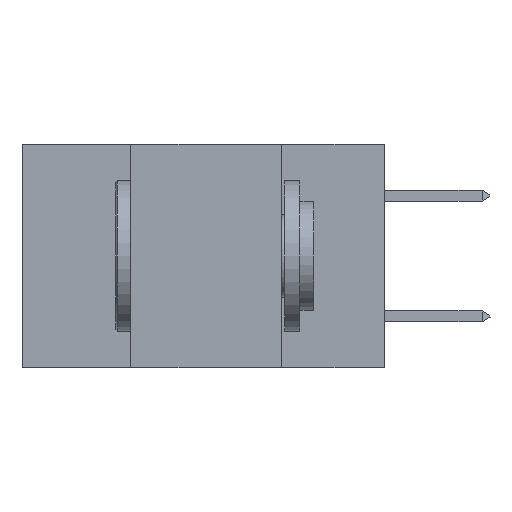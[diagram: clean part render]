
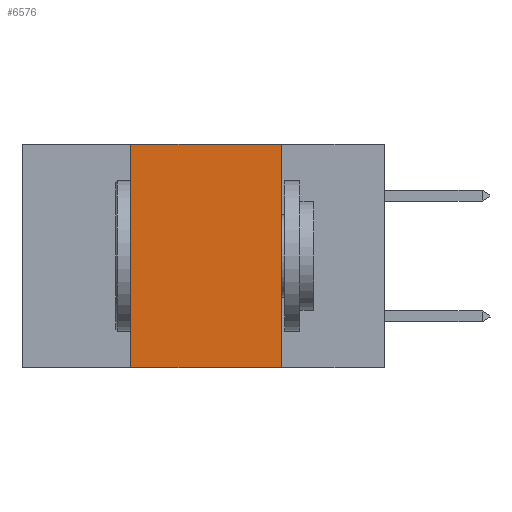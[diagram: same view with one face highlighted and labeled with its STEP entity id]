
A CAD part, left-side view. The second image highlights one B-rep face of the part: STEP entity #6576.
In plain terms, the highlighted planar face has unit normal (-1, 0, 0).
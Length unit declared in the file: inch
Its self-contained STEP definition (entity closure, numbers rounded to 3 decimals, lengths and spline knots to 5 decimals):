
#506 = VECTOR ( 'NONE', #9835, 39.37008 ) ;
#1009 = CARTESIAN_POINT ( 'NONE',  ( 0., 0.42, 0. ) ) ;
#1119 = EDGE_CURVE ( 'NONE', #10874, #10898, #22027, .T. ) ;
#1483 = DIRECTION ( 'NONE',  ( 0., -1., 0. ) ) ;
#1650 = EDGE_CURVE ( 'NONE', #10874, #3456, #13091, .T. ) ;
#2950 = CARTESIAN_POINT ( 'NONE',  ( 0., 0.6, -0.37 ) ) ;
#3456 = VERTEX_POINT ( 'NONE', #18937 ) ;
#4853 = LINE ( 'NONE', #17308, #19034 ) ;
#6576 = ADVANCED_FACE ( 'NONE', ( #27328 ), #13420, .F. ) ;
#6845 = VECTOR ( 'NONE', #17726, 39.37008 ) ;
#7116 = ORIENTED_EDGE ( 'NONE', *, *, #22655, .F. ) ;
#7169 = CARTESIAN_POINT ( 'NONE',  ( 0., 0.6, 0. ) ) ;
#9835 = DIRECTION ( 'NONE',  ( 0., -1., 0. ) ) ;
#9950 = DIRECTION ( 'NONE',  ( 1., 0., 0. ) ) ;
#10034 = DIRECTION ( 'NONE',  ( 0., 0., -1. ) ) ;
#10056 = VERTEX_POINT ( 'NONE', #16156 ) ;
#10874 = VERTEX_POINT ( 'NONE', #18403 ) ;
#10898 = VERTEX_POINT ( 'NONE', #20623 ) ;
#10921 = DIRECTION ( 'NONE',  ( 0., 0., -1. ) ) ;
#11898 = CARTESIAN_POINT ( 'NONE',  ( 0., 0.6, 0. ) ) ;
#12446 = EDGE_LOOP ( 'NONE', ( #7116, #24785, #25315, #26286 ) ) ;
#13091 = LINE ( 'NONE', #1009, #6845 ) ;
#13420 = PLANE ( 'NONE',  #26189 ) ;
#14283 = LINE ( 'NONE', #11898, #19868 ) ;
#16156 = CARTESIAN_POINT ( 'NONE',  ( 0., 0.17, 0. ) ) ;
#17308 = CARTESIAN_POINT ( 'NONE',  ( 0., 0.17, 0. ) ) ;
#17726 = DIRECTION ( 'NONE',  ( 0., 0., 1. ) ) ;
#18403 = CARTESIAN_POINT ( 'NONE',  ( 0., 0.42, -0.37 ) ) ;
#18937 = CARTESIAN_POINT ( 'NONE',  ( 0., 0.42, 0. ) ) ;
#19034 = VECTOR ( 'NONE', #10921, 39.37008 ) ;
#19652 = EDGE_CURVE ( 'NONE', #3456, #10056, #14283, .T. ) ;
#19868 = VECTOR ( 'NONE', #1483, 39.37008 ) ;
#20623 = CARTESIAN_POINT ( 'NONE',  ( 0., 0.17, -0.37 ) ) ;
#22027 = LINE ( 'NONE', #2950, #506 ) ;
#22655 = EDGE_CURVE ( 'NONE', #10056, #10898, #4853, .T. ) ;
#24785 = ORIENTED_EDGE ( 'NONE', *, *, #19652, .F. ) ;
#25315 = ORIENTED_EDGE ( 'NONE', *, *, #1650, .F. ) ;
#26189 = AXIS2_PLACEMENT_3D ( 'NONE', #7169, #9950, #10034 ) ;
#26286 = ORIENTED_EDGE ( 'NONE', *, *, #1119, .T. ) ;
#27328 = FACE_OUTER_BOUND ( 'NONE', #12446, .T. ) ;
